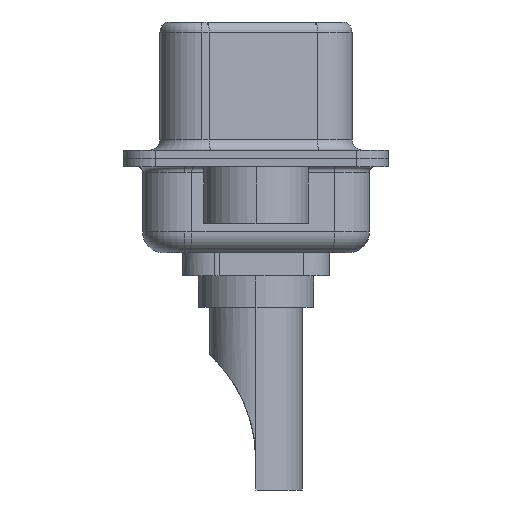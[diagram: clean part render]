
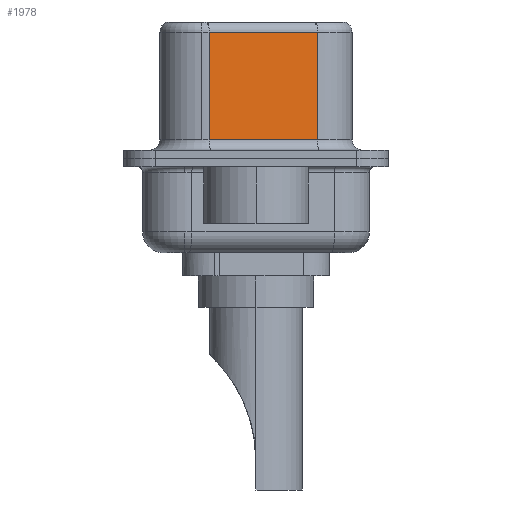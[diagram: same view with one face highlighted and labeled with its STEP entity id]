
A CAD part, left-side view. The second image highlights one B-rep face of the part: STEP entity #1978.
In plain terms, the highlighted planar face has unit normal (-0.985, -0.174, 0).
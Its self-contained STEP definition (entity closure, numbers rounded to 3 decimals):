
#1863 = ORIENTED_EDGE ( 'NONE', *, *, #14351, .F. ) ;
#1978 = ADVANCED_FACE ( 'NONE', ( #7497 ), #9968, .F. ) ;
#2071 = CARTESIAN_POINT ( 'NONE',  ( 3.67, 2.233, 0.9 ) ) ;
#2221 = CARTESIAN_POINT ( 'NONE',  ( 4.58, -2.927, 0.9 ) ) ;
#2820 = DIRECTION ( 'NONE',  ( -0.174, 0.985, 0. ) ) ;
#3011 = EDGE_LOOP ( 'NONE', ( #1863, #4424, #9322, #11214 ) ) ;
#3159 = VECTOR ( 'NONE', #7852, 1000. ) ;
#3776 = VERTEX_POINT ( 'NONE', #2071 ) ;
#4080 = LINE ( 'NONE', #7773, #9952 ) ;
#4424 = ORIENTED_EDGE ( 'NONE', *, *, #16136, .T. ) ;
#5009 = DIRECTION ( 'NONE',  ( 0.985, 0.174, 0. ) ) ;
#6689 = VECTOR ( 'NONE', #13213, 1000. ) ;
#6692 = CARTESIAN_POINT ( 'NONE',  ( 3.67, 2.233, 6.02 ) ) ;
#7405 = DIRECTION ( 'NONE',  ( -0.174, 0.985, 0. ) ) ;
#7497 = FACE_OUTER_BOUND ( 'NONE', #3011, .T. ) ;
#7773 = CARTESIAN_POINT ( 'NONE',  ( 4.58, -2.927, 0.9 ) ) ;
#7819 = VERTEX_POINT ( 'NONE', #12057 ) ;
#7852 = DIRECTION ( 'NONE',  ( 0., 0., -1. ) ) ;
#8212 = VERTEX_POINT ( 'NONE', #6692 ) ;
#9322 = ORIENTED_EDGE ( 'NONE', *, *, #13680, .T. ) ;
#9952 = VECTOR ( 'NONE', #15423, 1000. ) ;
#9968 = PLANE ( 'NONE',  #13950 ) ;
#10139 = VECTOR ( 'NONE', #2820, 1000. ) ;
#10682 = CARTESIAN_POINT ( 'NONE',  ( 4.58, -2.927, 6.52 ) ) ;
#11214 = ORIENTED_EDGE ( 'NONE', *, *, #11415, .T. ) ;
#11415 = EDGE_CURVE ( 'NONE', #3776, #14435, #4080, .T. ) ;
#11508 = CARTESIAN_POINT ( 'NONE',  ( 3.67, 2.233, 6.52 ) ) ;
#11526 = LINE ( 'NONE', #13040, #10139 ) ;
#11594 = LINE ( 'NONE', #11508, #3159 ) ;
#12057 = CARTESIAN_POINT ( 'NONE',  ( 4.58, -2.927, 6.02 ) ) ;
#13040 = CARTESIAN_POINT ( 'NONE',  ( 4.58, -2.927, 6.02 ) ) ;
#13213 = DIRECTION ( 'NONE',  ( 0., 0., -1. ) ) ;
#13680 = EDGE_CURVE ( 'NONE', #8212, #3776, #11594, .T. ) ;
#13950 = AXIS2_PLACEMENT_3D ( 'NONE', #14842, #5009, #7405 ) ;
#14351 = EDGE_CURVE ( 'NONE', #7819, #14435, #14540, .T. ) ;
#14435 = VERTEX_POINT ( 'NONE', #2221 ) ;
#14540 = LINE ( 'NONE', #10682, #6689 ) ;
#14842 = CARTESIAN_POINT ( 'NONE',  ( 4.58, -2.927, 6.52 ) ) ;
#15423 = DIRECTION ( 'NONE',  ( 0.174, -0.985, 0. ) ) ;
#16136 = EDGE_CURVE ( 'NONE', #7819, #8212, #11526, .T. ) ;
